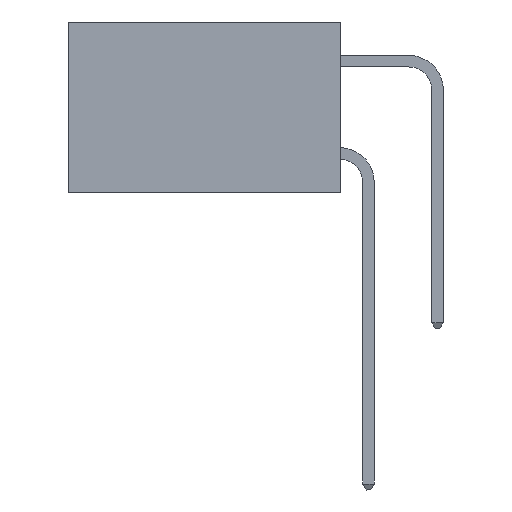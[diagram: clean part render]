
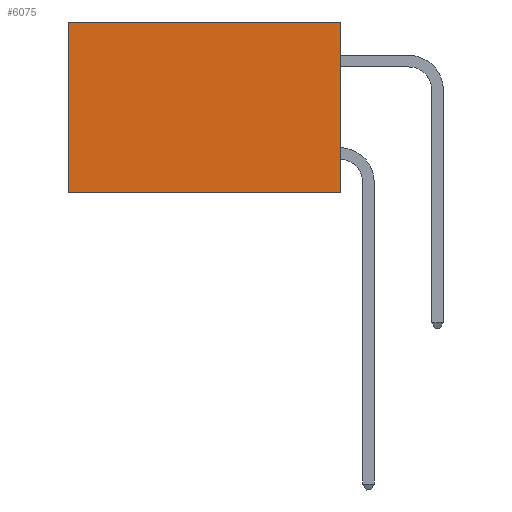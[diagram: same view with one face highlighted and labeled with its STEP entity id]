
A CAD part, left-side view. The second image highlights one B-rep face of the part: STEP entity #6075.
In plain terms, the highlighted planar face has unit normal (-1, 0, 0).
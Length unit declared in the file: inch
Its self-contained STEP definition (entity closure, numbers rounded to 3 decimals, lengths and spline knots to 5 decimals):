
#49 = EDGE_LOOP ( 'NONE', ( #13443, #10786, #8134, #8506 ) ) ;
#154 = CARTESIAN_POINT ( 'NONE',  ( 0.277, 0.59, -0.37 ) ) ;
#515 = VERTEX_POINT ( 'NONE', #12324 ) ;
#690 = VECTOR ( 'NONE', #13972, 39.37008 ) ;
#828 = DIRECTION ( 'NONE',  ( 0., 1., 0. ) ) ;
#830 = FACE_OUTER_BOUND ( 'NONE', #49, .T. ) ;
#2231 = DIRECTION ( 'NONE',  ( 0., 0., -1. ) ) ;
#2244 = DIRECTION ( 'NONE',  ( 1., 0., 0. ) ) ;
#2261 = CARTESIAN_POINT ( 'NONE',  ( 0.277, 0., -0.37 ) ) ;
#2312 = PLANE ( 'NONE',  #3375 ) ;
#2928 = EDGE_CURVE ( 'NONE', #7422, #12444, #11394, .T. ) ;
#3375 = AXIS2_PLACEMENT_3D ( 'NONE', #2261, #2244, #2231 ) ;
#4245 = EDGE_CURVE ( 'NONE', #7256, #12444, #9649, .T. ) ;
#4560 = VECTOR ( 'NONE', #12601, 39.37008 ) ;
#4727 = CARTESIAN_POINT ( 'NONE',  ( 0.277, 0.59, 0. ) ) ;
#5829 = CARTESIAN_POINT ( 'NONE',  ( 0.277, 0., -0.37 ) ) ;
#6075 = ADVANCED_FACE ( 'NONE', ( #830 ), #2312, .F. ) ;
#6143 = CARTESIAN_POINT ( 'NONE',  ( 0.277, 0., -0.37 ) ) ;
#7256 = VERTEX_POINT ( 'NONE', #6143 ) ;
#7422 = VERTEX_POINT ( 'NONE', #4727 ) ;
#8091 = DIRECTION ( 'NONE',  ( 0., 0., -1. ) ) ;
#8134 = ORIENTED_EDGE ( 'NONE', *, *, #13033, .F. ) ;
#8411 = VECTOR ( 'NONE', #8091, 39.37008 ) ;
#8506 = ORIENTED_EDGE ( 'NONE', *, *, #13388, .T. ) ;
#8690 = CARTESIAN_POINT ( 'NONE',  ( 0.277, 0., 0. ) ) ;
#8938 = VECTOR ( 'NONE', #828, 39.37008 ) ;
#8990 = CARTESIAN_POINT ( 'NONE',  ( 0.277, 0.59, -0.37 ) ) ;
#9649 = LINE ( 'NONE', #14051, #690 ) ;
#10786 = ORIENTED_EDGE ( 'NONE', *, *, #4245, .F. ) ;
#11394 = LINE ( 'NONE', #8990, #8411 ) ;
#11968 = LINE ( 'NONE', #8690, #8938 ) ;
#12324 = CARTESIAN_POINT ( 'NONE',  ( 0.277, 0., 0. ) ) ;
#12444 = VERTEX_POINT ( 'NONE', #154 ) ;
#12601 = DIRECTION ( 'NONE',  ( 0., 0., -1. ) ) ;
#13033 = EDGE_CURVE ( 'NONE', #515, #7256, #13541, .T. ) ;
#13388 = EDGE_CURVE ( 'NONE', #515, #7422, #11968, .T. ) ;
#13443 = ORIENTED_EDGE ( 'NONE', *, *, #2928, .T. ) ;
#13541 = LINE ( 'NONE', #5829, #4560 ) ;
#13972 = DIRECTION ( 'NONE',  ( 0., 1., 0. ) ) ;
#14051 = CARTESIAN_POINT ( 'NONE',  ( 0.277, 0., -0.37 ) ) ;
